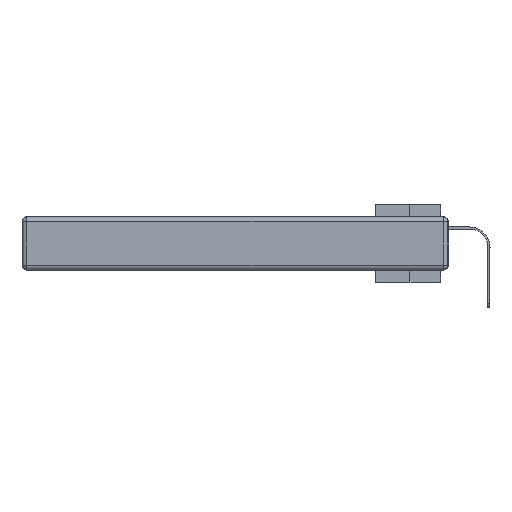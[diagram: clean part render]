
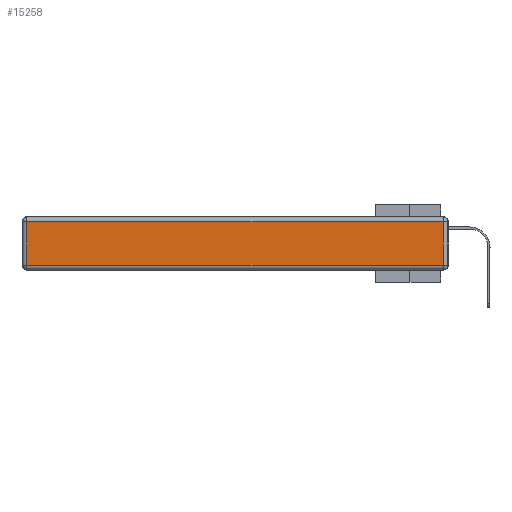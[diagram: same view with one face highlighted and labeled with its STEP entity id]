
A CAD part, left-side view. The second image highlights one B-rep face of the part: STEP entity #15258.
In plain terms, the highlighted planar face has unit normal (-1, 0, 0).
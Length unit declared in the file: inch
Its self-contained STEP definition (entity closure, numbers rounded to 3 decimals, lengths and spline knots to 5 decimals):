
#66 = PLANE ( 'NONE',  #11552 ) ;
#1541 = EDGE_CURVE ( 'NONE', #5564, #18906, #10412, .T. ) ;
#1758 = CARTESIAN_POINT ( 'NONE',  ( 0., 2.72, -0.343 ) ) ;
#2138 = DIRECTION ( 'NONE',  ( 0., -1., 0. ) ) ;
#2457 = CARTESIAN_POINT ( 'NONE',  ( 0., 0.03, -0.343 ) ) ;
#3703 = VERTEX_POINT ( 'NONE', #13920 ) ;
#5564 = VERTEX_POINT ( 'NONE', #20699 ) ;
#6180 = CARTESIAN_POINT ( 'NONE',  ( 0., 0., -0.313 ) ) ;
#8636 = CARTESIAN_POINT ( 'NONE',  ( 0., 0.03, -0.313 ) ) ;
#10412 = LINE ( 'NONE', #6180, #19072 ) ;
#10622 = CARTESIAN_POINT ( 'NONE',  ( 0., 2.72, -0.03 ) ) ;
#11552 = AXIS2_PLACEMENT_3D ( 'NONE', #22070, #23660, #21643 ) ;
#11952 = EDGE_CURVE ( 'NONE', #18906, #3703, #22156, .T. ) ;
#12704 = CARTESIAN_POINT ( 'NONE',  ( 0., 2.75, -0.03 ) ) ;
#13413 = VECTOR ( 'NONE', #23773, 39.37008 ) ;
#13920 = CARTESIAN_POINT ( 'NONE',  ( 0., 0.03, -0.03 ) ) ;
#14856 = EDGE_CURVE ( 'NONE', #3703, #20539, #28479, .T. ) ;
#15016 = DIRECTION ( 'NONE',  ( 0., 1., 0. ) ) ;
#15258 = ADVANCED_FACE ( 'NONE', ( #28290 ), #66, .T. ) ;
#15377 = LINE ( 'NONE', #1758, #13413 ) ;
#15642 = DIRECTION ( 'NONE',  ( 0., 0., 1. ) ) ;
#16838 = EDGE_CURVE ( 'NONE', #20539, #5564, #15377, .T. ) ;
#18547 = ORIENTED_EDGE ( 'NONE', *, *, #1541, .T. ) ;
#18906 = VERTEX_POINT ( 'NONE', #8636 ) ;
#19072 = VECTOR ( 'NONE', #2138, 39.37008 ) ;
#20170 = ORIENTED_EDGE ( 'NONE', *, *, #16838, .T. ) ;
#20539 = VERTEX_POINT ( 'NONE', #10622 ) ;
#20699 = CARTESIAN_POINT ( 'NONE',  ( 0., 2.72, -0.313 ) ) ;
#21028 = VECTOR ( 'NONE', #15642, 39.37008 ) ;
#21643 = DIRECTION ( 'NONE',  ( 0., 0., 1. ) ) ;
#22070 = CARTESIAN_POINT ( 'NONE',  ( 0., 0., -0.343 ) ) ;
#22156 = LINE ( 'NONE', #2457, #21028 ) ;
#23660 = DIRECTION ( 'NONE',  ( -1., 0., 0. ) ) ;
#23773 = DIRECTION ( 'NONE',  ( 0., 0., -1. ) ) ;
#24118 = VECTOR ( 'NONE', #15016, 39.37008 ) ;
#24533 = EDGE_LOOP ( 'NONE', ( #18547, #25291, #27647, #20170 ) ) ;
#25291 = ORIENTED_EDGE ( 'NONE', *, *, #11952, .T. ) ;
#27647 = ORIENTED_EDGE ( 'NONE', *, *, #14856, .T. ) ;
#28290 = FACE_OUTER_BOUND ( 'NONE', #24533, .T. ) ;
#28479 = LINE ( 'NONE', #12704, #24118 ) ;
